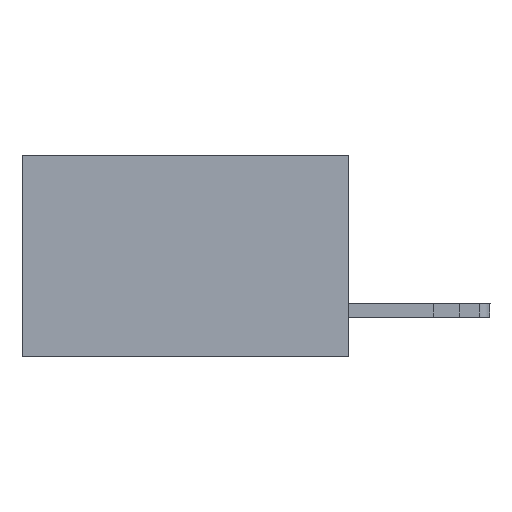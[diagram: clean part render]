
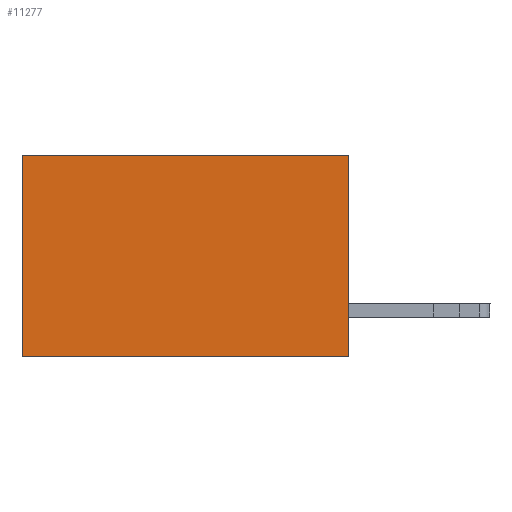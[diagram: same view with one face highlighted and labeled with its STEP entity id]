
A CAD part, left-side view. The second image highlights one B-rep face of the part: STEP entity #11277.
In plain terms, the highlighted planar face has unit normal (-1, 0, 0).
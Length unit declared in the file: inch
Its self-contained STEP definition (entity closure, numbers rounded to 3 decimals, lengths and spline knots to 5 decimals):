
#354 = DIRECTION ( 'NONE',  ( 1., 0., 0. ) ) ;
#1063 = LINE ( 'NONE', #4480, #11249 ) ;
#2538 = CARTESIAN_POINT ( 'NONE',  ( 0.298, 0.6, 0. ) ) ;
#3560 = CARTESIAN_POINT ( 'NONE',  ( 0.298, 0., 0. ) ) ;
#3627 = EDGE_CURVE ( 'NONE', #20410, #18533, #18527, .T. ) ;
#3887 = AXIS2_PLACEMENT_3D ( 'NONE', #13181, #354, #12778 ) ;
#4236 = ORIENTED_EDGE ( 'NONE', *, *, #13249, .T. ) ;
#4480 = CARTESIAN_POINT ( 'NONE',  ( 0.298, 0., 0. ) ) ;
#4930 = VECTOR ( 'NONE', #7281, 39.37008 ) ;
#5015 = ORIENTED_EDGE ( 'NONE', *, *, #3627, .F. ) ;
#6602 = ORIENTED_EDGE ( 'NONE', *, *, #16349, .F. ) ;
#6614 = ORIENTED_EDGE ( 'NONE', *, *, #14923, .T. ) ;
#6936 = EDGE_LOOP ( 'NONE', ( #4236, #6602, #5015, #6614 ) ) ;
#7281 = DIRECTION ( 'NONE',  ( 0., 0., -1. ) ) ;
#9147 = CARTESIAN_POINT ( 'NONE',  ( 0.298, 0.6, 0. ) ) ;
#9803 = VERTEX_POINT ( 'NONE', #9147 ) ;
#9880 = VECTOR ( 'NONE', #18630, 39.37008 ) ;
#10219 = VECTOR ( 'NONE', #17554, 39.37008 ) ;
#11249 = VECTOR ( 'NONE', #16787, 39.37008 ) ;
#11277 = ADVANCED_FACE ( 'NONE', ( #11613 ), #19186, .F. ) ;
#11613 = FACE_OUTER_BOUND ( 'NONE', #6936, .T. ) ;
#12778 = DIRECTION ( 'NONE',  ( 0., 0., -1. ) ) ;
#13181 = CARTESIAN_POINT ( 'NONE',  ( 0.298, 0., 0. ) ) ;
#13249 = EDGE_CURVE ( 'NONE', #9803, #19323, #18261, .T. ) ;
#13455 = CARTESIAN_POINT ( 'NONE',  ( 0.298, 0., -0.37 ) ) ;
#13981 = CARTESIAN_POINT ( 'NONE',  ( 0.298, 0., 0. ) ) ;
#14538 = CARTESIAN_POINT ( 'NONE',  ( 0.298, 0., -0.37 ) ) ;
#14826 = CARTESIAN_POINT ( 'NONE',  ( 0.298, 0.6, -0.37 ) ) ;
#14923 = EDGE_CURVE ( 'NONE', #20410, #9803, #1063, .T. ) ;
#16349 = EDGE_CURVE ( 'NONE', #18533, #19323, #19495, .T. ) ;
#16787 = DIRECTION ( 'NONE',  ( 0., 1., 0. ) ) ;
#17554 = DIRECTION ( 'NONE',  ( 0., 1., 0. ) ) ;
#18261 = LINE ( 'NONE', #2538, #4930 ) ;
#18527 = LINE ( 'NONE', #13981, #9880 ) ;
#18533 = VERTEX_POINT ( 'NONE', #13455 ) ;
#18630 = DIRECTION ( 'NONE',  ( 0., 0., -1. ) ) ;
#19186 = PLANE ( 'NONE',  #3887 ) ;
#19323 = VERTEX_POINT ( 'NONE', #14826 ) ;
#19495 = LINE ( 'NONE', #14538, #10219 ) ;
#20410 = VERTEX_POINT ( 'NONE', #3560 ) ;
